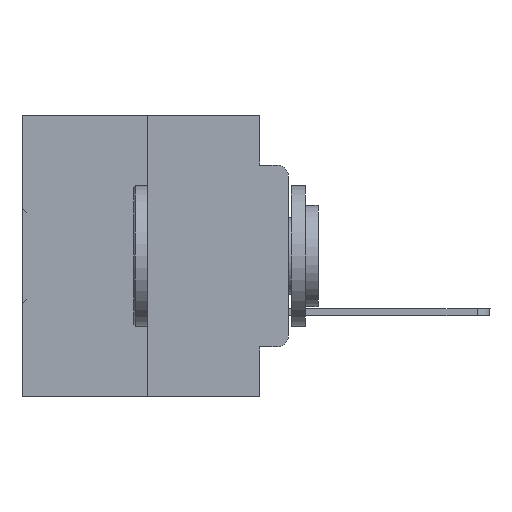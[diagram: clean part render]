
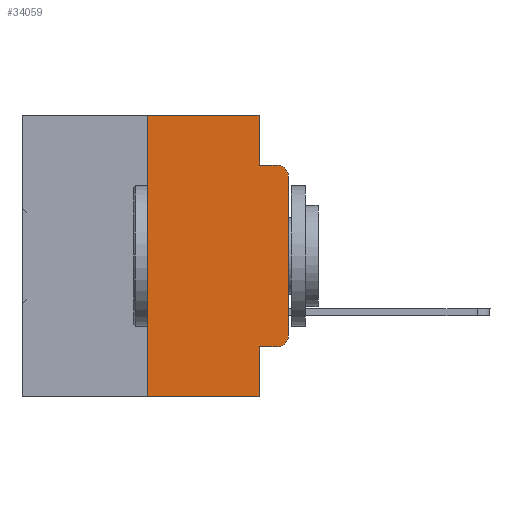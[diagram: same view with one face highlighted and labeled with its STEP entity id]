
A CAD part, left-side view. The second image highlights one B-rep face of the part: STEP entity #34059.
In plain terms, the highlighted planar face has unit normal (-1, 0, 0).
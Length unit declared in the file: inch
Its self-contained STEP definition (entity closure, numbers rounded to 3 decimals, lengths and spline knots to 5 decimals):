
#77 = ORIENTED_EDGE ( 'NONE', *, *, #22374, .F. ) ;
#770 = VERTEX_POINT ( 'NONE', #1794 ) ;
#949 = ORIENTED_EDGE ( 'NONE', *, *, #15593, .F. ) ;
#972 = EDGE_CURVE ( 'NONE', #8694, #13624, #22272, .T. ) ;
#1061 = DIRECTION ( 'NONE',  ( 0., -1., 0. ) ) ;
#1069 = EDGE_CURVE ( 'NONE', #770, #29314, #14172, .T. ) ;
#1384 = VERTEX_POINT ( 'NONE', #11398 ) ;
#1456 = LINE ( 'NONE', #4179, #24228 ) ;
#1794 = CARTESIAN_POINT ( 'NONE',  ( 0., 0.25, -0.5 ) ) ;
#1921 = VECTOR ( 'NONE', #12152, 39.37008 ) ;
#2268 = EDGE_CURVE ( 'NONE', #13624, #23146, #8855, .T. ) ;
#2848 = AXIS2_PLACEMENT_3D ( 'NONE', #6785, #4096, #12721 ) ;
#3242 = VECTOR ( 'NONE', #34603, 39.37008 ) ;
#3333 = DIRECTION ( 'NONE',  ( -1., 0., 0. ) ) ;
#3616 = CIRCLE ( 'NONE', #17981, 0.02 ) ;
#4035 = ORIENTED_EDGE ( 'NONE', *, *, #7695, .T. ) ;
#4096 = DIRECTION ( 'NONE',  ( 1., 0., 0. ) ) ;
#4179 = CARTESIAN_POINT ( 'NONE',  ( 0., 0.051, 0. ) ) ;
#4543 = CARTESIAN_POINT ( 'NONE',  ( 0., 0., 0. ) ) ;
#4736 = CARTESIAN_POINT ( 'NONE',  ( 0., 0.473, 0. ) ) ;
#5644 = CARTESIAN_POINT ( 'NONE',  ( 0., 0.051, -0.4115 ) ) ;
#6785 = CARTESIAN_POINT ( 'NONE',  ( 0., 0.473, 0. ) ) ;
#7329 = VERTEX_POINT ( 'NONE', #8171 ) ;
#7682 = VECTOR ( 'NONE', #34464, 39.37008 ) ;
#7695 = EDGE_CURVE ( 'NONE', #18674, #1384, #3616, .T. ) ;
#8171 = CARTESIAN_POINT ( 'NONE',  ( 0., 0.051, -0.0885 ) ) ;
#8284 = CARTESIAN_POINT ( 'NONE',  ( 0., 0.051, 0. ) ) ;
#8367 = DIRECTION ( 'NONE',  ( 0., 0., -1. ) ) ;
#8426 = CARTESIAN_POINT ( 'NONE',  ( 0., 0.051, -0.4115 ) ) ;
#8694 = VERTEX_POINT ( 'NONE', #5644 ) ;
#8855 = CIRCLE ( 'NONE', #27250, 0.02 ) ;
#9400 = DIRECTION ( 'NONE',  ( 0., 0., -1. ) ) ;
#9557 = CARTESIAN_POINT ( 'NONE',  ( 0., 0.473, -0.5 ) ) ;
#9593 = LINE ( 'NONE', #4736, #3242 ) ;
#11398 = CARTESIAN_POINT ( 'NONE',  ( 0., 0.02, -0.0885 ) ) ;
#11777 = EDGE_LOOP ( 'NONE', ( #14482, #4035, #77, #22800, #949, #35291, #18577, #16118, #32126, #26382 ) ) ;
#12152 = DIRECTION ( 'NONE',  ( 0., -1., 0. ) ) ;
#12721 = DIRECTION ( 'NONE',  ( 0., 0., -1. ) ) ;
#13624 = VERTEX_POINT ( 'NONE', #18693 ) ;
#14172 = LINE ( 'NONE', #25149, #7682 ) ;
#14482 = ORIENTED_EDGE ( 'NONE', *, *, #30694, .T. ) ;
#14699 = PLANE ( 'NONE',  #2848 ) ;
#15115 = LINE ( 'NONE', #20686, #22251 ) ;
#15593 = EDGE_CURVE ( 'NONE', #29314, #22254, #9593, .T. ) ;
#15612 = VECTOR ( 'NONE', #20905, 39.37008 ) ;
#16118 = ORIENTED_EDGE ( 'NONE', *, *, #34372, .F. ) ;
#16463 = LINE ( 'NONE', #33014, #19553 ) ;
#16595 = CARTESIAN_POINT ( 'NONE',  ( 0., 0.25, 0. ) ) ;
#16866 = CARTESIAN_POINT ( 'NONE',  ( 0., 0., -0.3915 ) ) ;
#17286 = EDGE_CURVE ( 'NONE', #770, #35582, #18551, .T. ) ;
#17981 = AXIS2_PLACEMENT_3D ( 'NONE', #27027, #18409, #23806 ) ;
#18409 = DIRECTION ( 'NONE',  ( -1., 0., 0. ) ) ;
#18551 = LINE ( 'NONE', #9557, #15612 ) ;
#18577 = ORIENTED_EDGE ( 'NONE', *, *, #17286, .T. ) ;
#18674 = VERTEX_POINT ( 'NONE', #28721 ) ;
#18693 = CARTESIAN_POINT ( 'NONE',  ( 0., 0.02, -0.4115 ) ) ;
#18752 = CARTESIAN_POINT ( 'NONE',  ( 0., 0.051, -0.5 ) ) ;
#19553 = VECTOR ( 'NONE', #8367, 39.37008 ) ;
#20686 = CARTESIAN_POINT ( 'NONE',  ( 0., 0.051, -0.0885 ) ) ;
#20775 = EDGE_CURVE ( 'NONE', #22254, #7329, #1456, .T. ) ;
#20905 = DIRECTION ( 'NONE',  ( 0., -1., 0. ) ) ;
#22251 = VECTOR ( 'NONE', #1061, 39.37008 ) ;
#22254 = VERTEX_POINT ( 'NONE', #8284 ) ;
#22272 = LINE ( 'NONE', #8426, #1921 ) ;
#22374 = EDGE_CURVE ( 'NONE', #7329, #1384, #15115, .T. ) ;
#22800 = ORIENTED_EDGE ( 'NONE', *, *, #20775, .F. ) ;
#23146 = VERTEX_POINT ( 'NONE', #16866 ) ;
#23806 = DIRECTION ( 'NONE',  ( 0., 0., -1. ) ) ;
#24228 = VECTOR ( 'NONE', #9400, 39.37008 ) ;
#25149 = CARTESIAN_POINT ( 'NONE',  ( 0., 0.25, 0. ) ) ;
#26382 = ORIENTED_EDGE ( 'NONE', *, *, #2268, .T. ) ;
#26496 = DIRECTION ( 'NONE',  ( 0., 0., 1. ) ) ;
#27027 = CARTESIAN_POINT ( 'NONE',  ( 0., 0.02, -0.1085 ) ) ;
#27250 = AXIS2_PLACEMENT_3D ( 'NONE', #27994, #3333, #33742 ) ;
#27994 = CARTESIAN_POINT ( 'NONE',  ( 0., 0.02, -0.3915 ) ) ;
#28254 = VECTOR ( 'NONE', #26496, 39.37008 ) ;
#28721 = CARTESIAN_POINT ( 'NONE',  ( 0., 0., -0.1085 ) ) ;
#28846 = LINE ( 'NONE', #4543, #28254 ) ;
#29314 = VERTEX_POINT ( 'NONE', #16595 ) ;
#30694 = EDGE_CURVE ( 'NONE', #23146, #18674, #28846, .T. ) ;
#31800 = FACE_OUTER_BOUND ( 'NONE', #11777, .T. ) ;
#32126 = ORIENTED_EDGE ( 'NONE', *, *, #972, .T. ) ;
#33014 = CARTESIAN_POINT ( 'NONE',  ( 0., 0.051, 0. ) ) ;
#33742 = DIRECTION ( 'NONE',  ( 0., 0., -1. ) ) ;
#34059 = ADVANCED_FACE ( 'NONE', ( #31800 ), #14699, .F. ) ;
#34372 = EDGE_CURVE ( 'NONE', #8694, #35582, #16463, .T. ) ;
#34464 = DIRECTION ( 'NONE',  ( 0., 0., 1. ) ) ;
#34603 = DIRECTION ( 'NONE',  ( 0., -1., 0. ) ) ;
#35291 = ORIENTED_EDGE ( 'NONE', *, *, #1069, .F. ) ;
#35582 = VERTEX_POINT ( 'NONE', #18752 ) ;
